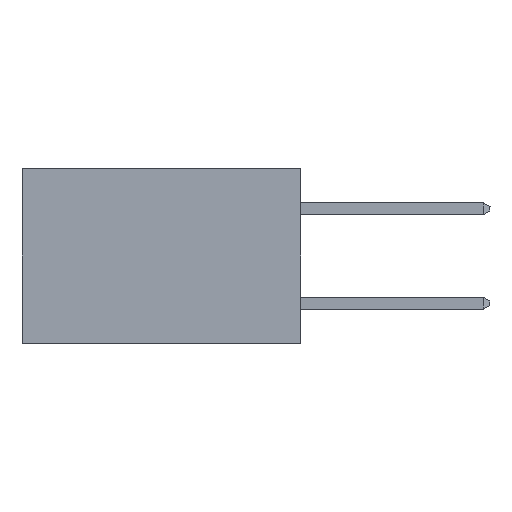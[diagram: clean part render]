
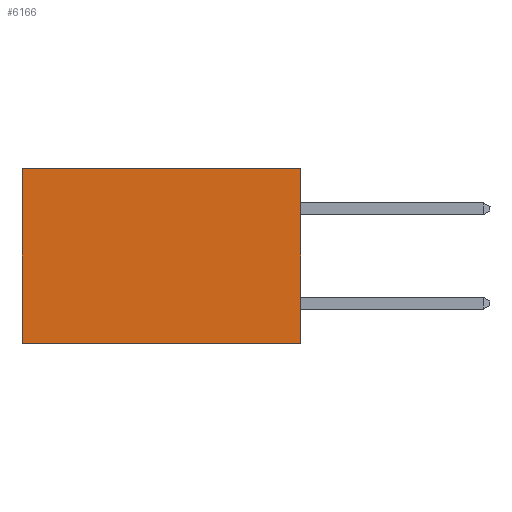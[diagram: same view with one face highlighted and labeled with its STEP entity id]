
A CAD part, left-side view. The second image highlights one B-rep face of the part: STEP entity #6166.
In plain terms, the highlighted planar face has unit normal (-1, 0, 0).
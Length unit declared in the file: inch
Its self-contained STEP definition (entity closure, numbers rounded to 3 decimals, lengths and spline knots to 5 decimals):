
#742 = DIRECTION ( 'NONE',  ( 0., 0., -1. ) ) ;
#887 = ORIENTED_EDGE ( 'NONE', *, *, #8309, .T. ) ;
#1164 = VERTEX_POINT ( 'NONE', #6617 ) ;
#1736 = CARTESIAN_POINT ( 'NONE',  ( 0.277, 0.59, -0.37 ) ) ;
#2013 = ORIENTED_EDGE ( 'NONE', *, *, #9353, .F. ) ;
#2156 = LINE ( 'NONE', #8067, #5120 ) ;
#2270 = VERTEX_POINT ( 'NONE', #4853 ) ;
#2549 = CARTESIAN_POINT ( 'NONE',  ( 0.277, 0., -0.37 ) ) ;
#3332 = CARTESIAN_POINT ( 'NONE',  ( 0.277, 0.59, 0. ) ) ;
#3345 = AXIS2_PLACEMENT_3D ( 'NONE', #6887, #6872, #6838 ) ;
#3947 = CARTESIAN_POINT ( 'NONE',  ( 0.277, 0., 0. ) ) ;
#4431 = FACE_OUTER_BOUND ( 'NONE', #6868, .T. ) ;
#4853 = CARTESIAN_POINT ( 'NONE',  ( 0.277, 0., 0. ) ) ;
#5120 = VECTOR ( 'NONE', #10701, 39.37008 ) ;
#5272 = LINE ( 'NONE', #3947, #7717 ) ;
#5726 = EDGE_CURVE ( 'NONE', #10298, #1164, #11701, .T. ) ;
#6166 = ADVANCED_FACE ( 'NONE', ( #4431 ), #6905, .F. ) ;
#6617 = CARTESIAN_POINT ( 'NONE',  ( 0.277, 0.59, -0.37 ) ) ;
#6838 = DIRECTION ( 'NONE',  ( 0., 0., -1. ) ) ;
#6868 = EDGE_LOOP ( 'NONE', ( #8255, #2013, #9398, #887 ) ) ;
#6872 = DIRECTION ( 'NONE',  ( 1., 0., 0. ) ) ;
#6887 = CARTESIAN_POINT ( 'NONE',  ( 0.277, 0., -0.37 ) ) ;
#6905 = PLANE ( 'NONE',  #3345 ) ;
#7519 = VERTEX_POINT ( 'NONE', #2549 ) ;
#7717 = VECTOR ( 'NONE', #11209, 39.37008 ) ;
#8067 = CARTESIAN_POINT ( 'NONE',  ( 0.277, 0., -0.37 ) ) ;
#8255 = ORIENTED_EDGE ( 'NONE', *, *, #5726, .T. ) ;
#8309 = EDGE_CURVE ( 'NONE', #2270, #10298, #5272, .T. ) ;
#8314 = CARTESIAN_POINT ( 'NONE',  ( 0.277, 0., -0.37 ) ) ;
#8385 = VECTOR ( 'NONE', #10112, 39.37008 ) ;
#8631 = EDGE_CURVE ( 'NONE', #2270, #7519, #2156, .T. ) ;
#9022 = VECTOR ( 'NONE', #742, 39.37008 ) ;
#9353 = EDGE_CURVE ( 'NONE', #7519, #1164, #10751, .T. ) ;
#9398 = ORIENTED_EDGE ( 'NONE', *, *, #8631, .F. ) ;
#10112 = DIRECTION ( 'NONE',  ( 0., 1., 0. ) ) ;
#10298 = VERTEX_POINT ( 'NONE', #3332 ) ;
#10701 = DIRECTION ( 'NONE',  ( 0., 0., -1. ) ) ;
#10751 = LINE ( 'NONE', #8314, #8385 ) ;
#11209 = DIRECTION ( 'NONE',  ( 0., 1., 0. ) ) ;
#11701 = LINE ( 'NONE', #1736, #9022 ) ;
